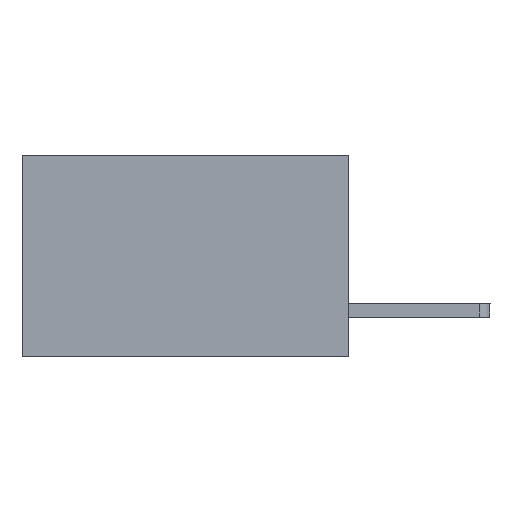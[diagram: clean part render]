
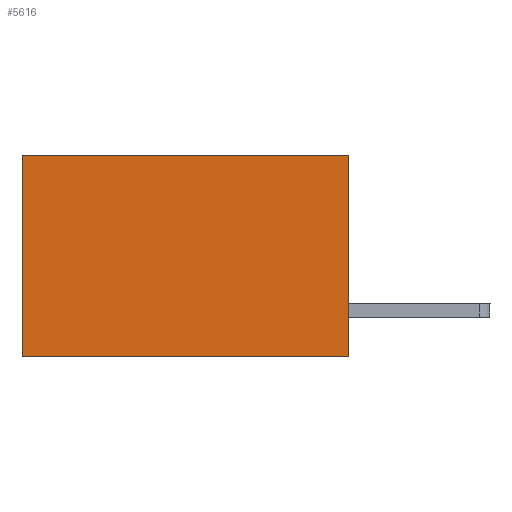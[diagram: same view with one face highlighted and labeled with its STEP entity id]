
A CAD part, left-side view. The second image highlights one B-rep face of the part: STEP entity #5616.
In plain terms, the highlighted planar face has unit normal (-1, 0, 0).
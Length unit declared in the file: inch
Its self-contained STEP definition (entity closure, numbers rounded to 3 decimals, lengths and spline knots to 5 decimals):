
#205 = VERTEX_POINT ( 'NONE', #4379 ) ;
#524 = DIRECTION ( 'NONE',  ( 1., 0., 0. ) ) ;
#1154 = EDGE_LOOP ( 'NONE', ( #6222, #7063, #1167, #1722 ) ) ;
#1163 = EDGE_CURVE ( 'NONE', #205, #9112, #5614, .T. ) ;
#1167 = ORIENTED_EDGE ( 'NONE', *, *, #6948, .F. ) ;
#1430 = VERTEX_POINT ( 'NONE', #6044 ) ;
#1722 = ORIENTED_EDGE ( 'NONE', *, *, #1163, .T. ) ;
#2026 = FACE_OUTER_BOUND ( 'NONE', #1154, .T. ) ;
#2302 = CARTESIAN_POINT ( 'NONE',  ( 0.2615, 0., -0.37 ) ) ;
#2957 = DIRECTION ( 'NONE',  ( 0., 1., 0. ) ) ;
#3417 = DIRECTION ( 'NONE',  ( 0., 0., -1. ) ) ;
#3742 = DIRECTION ( 'NONE',  ( 0., 0., -1. ) ) ;
#4372 = PLANE ( 'NONE',  #4426 ) ;
#4379 = CARTESIAN_POINT ( 'NONE',  ( 0.2615, 0., 0. ) ) ;
#4391 = LINE ( 'NONE', #6531, #5663 ) ;
#4396 = VECTOR ( 'NONE', #2957, 39.37008 ) ;
#4426 = AXIS2_PLACEMENT_3D ( 'NONE', #7423, #524, #3742 ) ;
#4756 = CARTESIAN_POINT ( 'NONE',  ( 0.2615, 0.6, -0.37 ) ) ;
#4966 = CARTESIAN_POINT ( 'NONE',  ( 0.2615, 0., 0. ) ) ;
#5077 = CARTESIAN_POINT ( 'NONE',  ( 0.2615, 0.6, 0. ) ) ;
#5614 = LINE ( 'NONE', #4966, #6363 ) ;
#5616 = ADVANCED_FACE ( 'NONE', ( #2026 ), #4372, .F. ) ;
#5663 = VECTOR ( 'NONE', #3417, 39.37008 ) ;
#6044 = CARTESIAN_POINT ( 'NONE',  ( 0.2615, 0., -0.37 ) ) ;
#6222 = ORIENTED_EDGE ( 'NONE', *, *, #9383, .T. ) ;
#6363 = VECTOR ( 'NONE', #7863, 39.37008 ) ;
#6399 = VERTEX_POINT ( 'NONE', #8468 ) ;
#6531 = CARTESIAN_POINT ( 'NONE',  ( 0.2615, 0., -0.37 ) ) ;
#6948 = EDGE_CURVE ( 'NONE', #205, #1430, #4391, .T. ) ;
#7058 = EDGE_CURVE ( 'NONE', #1430, #6399, #8336, .T. ) ;
#7063 = ORIENTED_EDGE ( 'NONE', *, *, #7058, .F. ) ;
#7110 = DIRECTION ( 'NONE',  ( 0., 0., -1. ) ) ;
#7423 = CARTESIAN_POINT ( 'NONE',  ( 0.2615, 0., -0.37 ) ) ;
#7667 = LINE ( 'NONE', #4756, #9241 ) ;
#7863 = DIRECTION ( 'NONE',  ( 0., 1., 0. ) ) ;
#8336 = LINE ( 'NONE', #2302, #4396 ) ;
#8468 = CARTESIAN_POINT ( 'NONE',  ( 0.2615, 0.6, -0.37 ) ) ;
#9112 = VERTEX_POINT ( 'NONE', #5077 ) ;
#9241 = VECTOR ( 'NONE', #7110, 39.37008 ) ;
#9383 = EDGE_CURVE ( 'NONE', #9112, #6399, #7667, .T. ) ;
